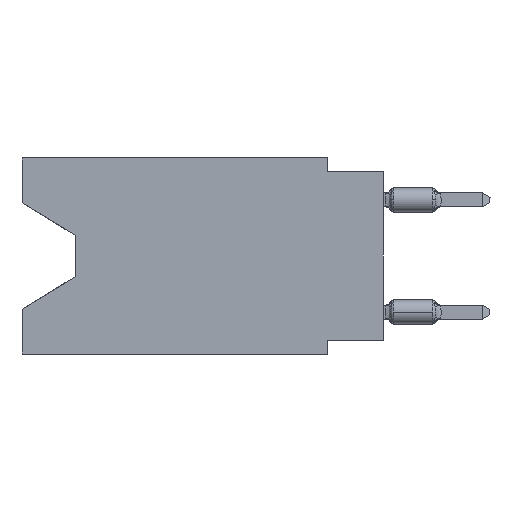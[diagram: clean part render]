
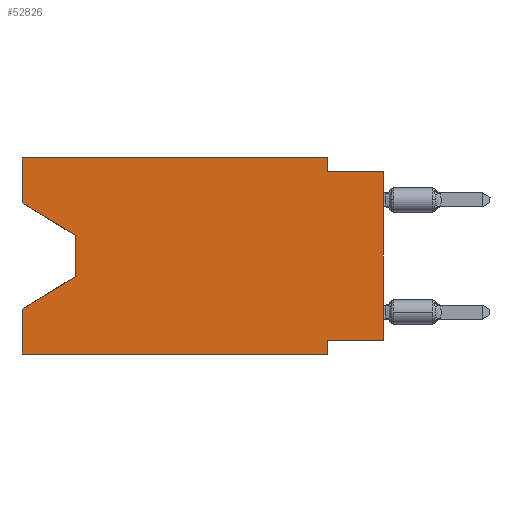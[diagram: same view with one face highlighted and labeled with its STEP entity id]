
A CAD part, left-side view. The second image highlights one B-rep face of the part: STEP entity #52826.
In plain terms, the highlighted planar face has unit normal (-1, 0, 0).
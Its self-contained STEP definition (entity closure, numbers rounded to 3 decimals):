
#34 = DIRECTION ( 'NONE',  ( 0., 0., -1. ) ) ;
#541 = EDGE_CURVE ( 'NONE', #6194, #21272, #53005, .T. ) ;
#1494 = CARTESIAN_POINT ( 'NONE',  ( 0., 16.383, 0. ) ) ;
#1734 = CARTESIAN_POINT ( 'NONE',  ( 0., 16.383, -2.038 ) ) ;
#2183 = CARTESIAN_POINT ( 'NONE',  ( 0., 0., 0. ) ) ;
#2362 = LINE ( 'NONE', #28072, #35739 ) ;
#3674 = EDGE_CURVE ( 'NONE', #34168, #24746, #42816, .T. ) ;
#5061 = LINE ( 'NONE', #17362, #15968 ) ;
#5092 = VERTEX_POINT ( 'NONE', #5907 ) ;
#5829 = LINE ( 'NONE', #9492, #50908 ) ;
#5886 = DIRECTION ( 'NONE',  ( 1., 0., 0. ) ) ;
#5907 = CARTESIAN_POINT ( 'NONE',  ( 0., 0., -0.635 ) ) ;
#6194 = VERTEX_POINT ( 'NONE', #9574 ) ;
#6334 = VERTEX_POINT ( 'NONE', #1734 ) ;
#6760 = ORIENTED_EDGE ( 'NONE', *, *, #3674, .T. ) ;
#6919 = DIRECTION ( 'NONE',  ( 0., 0., 1. ) ) ;
#7013 = ORIENTED_EDGE ( 'NONE', *, *, #16250, .T. ) ;
#8155 = CARTESIAN_POINT ( 'NONE',  ( 0., 0., -0.635 ) ) ;
#8222 = LINE ( 'NONE', #54361, #41779 ) ;
#9492 = CARTESIAN_POINT ( 'NONE',  ( 0., 13.97, -3.505 ) ) ;
#9574 = CARTESIAN_POINT ( 'NONE',  ( 0., 16.383, -8.89 ) ) ;
#10254 = CARTESIAN_POINT ( 'NONE',  ( 0., 13.97, -3.505 ) ) ;
#11107 = EDGE_CURVE ( 'NONE', #40979, #38035, #34312, .T. ) ;
#11399 = LINE ( 'NONE', #2183, #27924 ) ;
#12551 = EDGE_CURVE ( 'NONE', #44111, #34168, #5829, .T. ) ;
#14470 = DIRECTION ( 'NONE',  ( 0., 0., 1. ) ) ;
#14684 = EDGE_CURVE ( 'NONE', #33308, #22363, #2362, .T. ) ;
#14836 = CARTESIAN_POINT ( 'NONE',  ( 0., 16.383, 0. ) ) ;
#14944 = CARTESIAN_POINT ( 'NONE',  ( 0., 0., -8.255 ) ) ;
#15570 = CARTESIAN_POINT ( 'NONE',  ( 0., 16.383, 0. ) ) ;
#15968 = VECTOR ( 'NONE', #34, 1000. ) ;
#16250 = EDGE_CURVE ( 'NONE', #6334, #44111, #44249, .T. ) ;
#16401 = CARTESIAN_POINT ( 'NONE',  ( 0., 16.383, 0. ) ) ;
#16979 = ORIENTED_EDGE ( 'NONE', *, *, #31471, .F. ) ;
#17362 = CARTESIAN_POINT ( 'NONE',  ( 0., 2.54, 0. ) ) ;
#17437 = CARTESIAN_POINT ( 'NONE',  ( 0., 16.383, -6.852 ) ) ;
#18146 = DIRECTION ( 'NONE',  ( 0., 0., -1. ) ) ;
#20010 = ORIENTED_EDGE ( 'NONE', *, *, #33663, .T. ) ;
#20110 = ORIENTED_EDGE ( 'NONE', *, *, #49943, .F. ) ;
#20468 = VECTOR ( 'NONE', #41237, 1000. ) ;
#20801 = DIRECTION ( 'NONE',  ( 0., 0., -1. ) ) ;
#21272 = VERTEX_POINT ( 'NONE', #48728 ) ;
#21562 = DIRECTION ( 'NONE',  ( 0., -1., 0. ) ) ;
#21633 = CARTESIAN_POINT ( 'NONE',  ( 0., 2.54, -8.255 ) ) ;
#22363 = VERTEX_POINT ( 'NONE', #23975 ) ;
#22543 = ORIENTED_EDGE ( 'NONE', *, *, #12551, .T. ) ;
#22963 = ORIENTED_EDGE ( 'NONE', *, *, #541, .T. ) ;
#23496 = ORIENTED_EDGE ( 'NONE', *, *, #47655, .F. ) ;
#23975 = CARTESIAN_POINT ( 'NONE',  ( 0., 2.54, 0. ) ) ;
#24746 = VERTEX_POINT ( 'NONE', #17437 ) ;
#25645 = CARTESIAN_POINT ( 'NONE',  ( 0., 0., -8.255 ) ) ;
#26056 = DIRECTION ( 'NONE',  ( 0., 0.855, -0.519 ) ) ;
#26956 = ORIENTED_EDGE ( 'NONE', *, *, #49444, .F. ) ;
#26995 = VECTOR ( 'NONE', #26056, 1000. ) ;
#27393 = VECTOR ( 'NONE', #14470, 1000. ) ;
#27924 = VECTOR ( 'NONE', #6919, 1000. ) ;
#28072 = CARTESIAN_POINT ( 'NONE',  ( 0., 16.383, 0. ) ) ;
#29270 = LINE ( 'NONE', #16401, #40848 ) ;
#30679 = DIRECTION ( 'NONE',  ( 0., 1., 0. ) ) ;
#31471 = EDGE_CURVE ( 'NONE', #6194, #24746, #29270, .T. ) ;
#31680 = CARTESIAN_POINT ( 'NONE',  ( 0., 16.383, -2.038 ) ) ;
#31761 = EDGE_CURVE ( 'NONE', #39079, #5092, #46450, .T. ) ;
#33308 = VERTEX_POINT ( 'NONE', #1494 ) ;
#33461 = DIRECTION ( 'NONE',  ( 0., 0., 1. ) ) ;
#33663 = EDGE_CURVE ( 'NONE', #40979, #5092, #11399, .T. ) ;
#34161 = CARTESIAN_POINT ( 'NONE',  ( 0., 13.97, -5.385 ) ) ;
#34168 = VERTEX_POINT ( 'NONE', #36772 ) ;
#34312 = LINE ( 'NONE', #25645, #35650 ) ;
#35110 = AXIS2_PLACEMENT_3D ( 'NONE', #14836, #5886, #39174 ) ;
#35617 = ORIENTED_EDGE ( 'NONE', *, *, #11107, .F. ) ;
#35650 = VECTOR ( 'NONE', #30679, 1000. ) ;
#35739 = VECTOR ( 'NONE', #48476, 1000. ) ;
#35804 = PLANE ( 'NONE',  #35110 ) ;
#36772 = CARTESIAN_POINT ( 'NONE',  ( 0., 13.97, -5.385 ) ) ;
#38035 = VERTEX_POINT ( 'NONE', #21633 ) ;
#39079 = VERTEX_POINT ( 'NONE', #46828 ) ;
#39174 = DIRECTION ( 'NONE',  ( 0., 0., -1. ) ) ;
#40848 = VECTOR ( 'NONE', #33461, 1000. ) ;
#40979 = VERTEX_POINT ( 'NONE', #14944 ) ;
#41237 = DIRECTION ( 'NONE',  ( 0., -1., 0. ) ) ;
#41486 = VECTOR ( 'NONE', #44518, 1000. ) ;
#41779 = VECTOR ( 'NONE', #20801, 1000. ) ;
#42076 = EDGE_LOOP ( 'NONE', ( #7013, #22543, #6760, #16979, #22963, #26956, #35617, #20010, #43829, #20110, #50559, #23496 ) ) ;
#42816 = LINE ( 'NONE', #34161, #26995 ) ;
#43829 = ORIENTED_EDGE ( 'NONE', *, *, #31761, .F. ) ;
#44111 = VERTEX_POINT ( 'NONE', #10254 ) ;
#44249 = LINE ( 'NONE', #31680, #41486 ) ;
#44518 = DIRECTION ( 'NONE',  ( 0., -0.855, -0.519 ) ) ;
#45158 = CARTESIAN_POINT ( 'NONE',  ( 0., 16.383, -8.89 ) ) ;
#46450 = LINE ( 'NONE', #8155, #48946 ) ;
#46828 = CARTESIAN_POINT ( 'NONE',  ( 0., 2.54, -0.635 ) ) ;
#47655 = EDGE_CURVE ( 'NONE', #6334, #33308, #52766, .T. ) ;
#48476 = DIRECTION ( 'NONE',  ( 0., -1., 0. ) ) ;
#48728 = CARTESIAN_POINT ( 'NONE',  ( 0., 2.54, -8.89 ) ) ;
#48946 = VECTOR ( 'NONE', #21562, 1000. ) ;
#49444 = EDGE_CURVE ( 'NONE', #38035, #21272, #8222, .T. ) ;
#49943 = EDGE_CURVE ( 'NONE', #22363, #39079, #5061, .T. ) ;
#50559 = ORIENTED_EDGE ( 'NONE', *, *, #14684, .F. ) ;
#50908 = VECTOR ( 'NONE', #18146, 1000. ) ;
#52300 = FACE_OUTER_BOUND ( 'NONE', #42076, .T. ) ;
#52766 = LINE ( 'NONE', #15570, #27393 ) ;
#52826 = ADVANCED_FACE ( 'NONE', ( #52300 ), #35804, .F. ) ;
#53005 = LINE ( 'NONE', #45158, #20468 ) ;
#54361 = CARTESIAN_POINT ( 'NONE',  ( 0., 2.54, -8.89 ) ) ;
